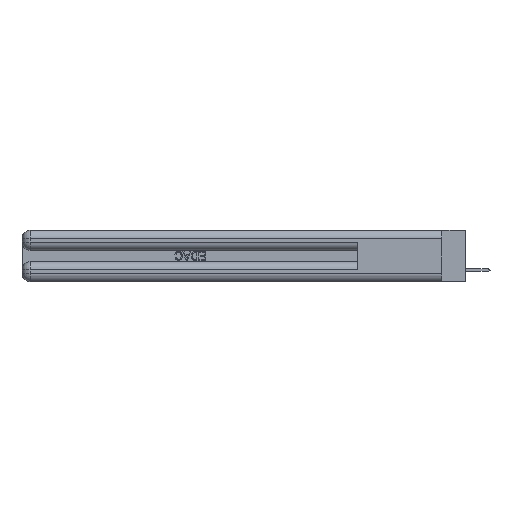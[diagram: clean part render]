
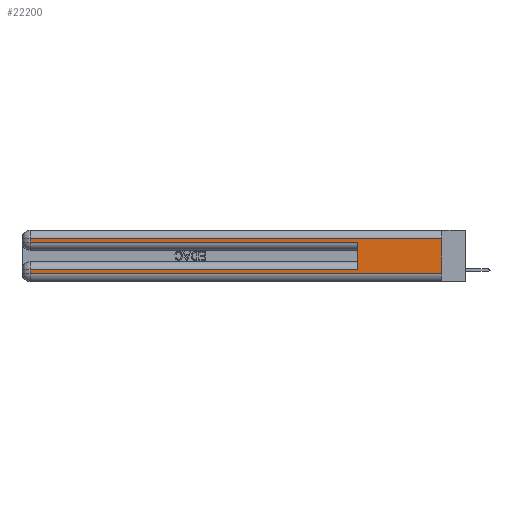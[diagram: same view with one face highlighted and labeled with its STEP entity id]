
A CAD part, left-side view. The second image highlights one B-rep face of the part: STEP entity #22200.
In plain terms, the highlighted planar face has unit normal (-1, 0, 0).
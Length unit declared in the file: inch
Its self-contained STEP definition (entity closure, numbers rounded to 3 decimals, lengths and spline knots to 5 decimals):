
#87 = EDGE_CURVE ( 'NONE', #17412, #18980, #23298, .T. ) ;
#393 = DIRECTION ( 'NONE',  ( 0., -1., 0. ) ) ;
#1524 = DIRECTION ( 'NONE',  ( 0., 0., -1. ) ) ;
#2635 = FACE_OUTER_BOUND ( 'NONE', #38131, .T. ) ;
#3554 = LINE ( 'NONE', #44252, #30137 ) ;
#4403 = LINE ( 'NONE', #26620, #36100 ) ;
#4473 = ORIENTED_EDGE ( 'NONE', *, *, #4612, .T. ) ;
#4612 = EDGE_CURVE ( 'NONE', #8973, #6380, #8666, .T. ) ;
#4940 = EDGE_CURVE ( 'NONE', #36621, #8973, #3554, .T. ) ;
#5644 = ORIENTED_EDGE ( 'NONE', *, *, #29355, .T. ) ;
#6380 = VERTEX_POINT ( 'NONE', #15923 ) ;
#6638 = LINE ( 'NONE', #37031, #34373 ) ;
#8666 = LINE ( 'NONE', #25550, #30186 ) ;
#8712 = ORIENTED_EDGE ( 'NONE', *, *, #26501, .T. ) ;
#8973 = VERTEX_POINT ( 'NONE', #36104 ) ;
#9249 = VERTEX_POINT ( 'NONE', #35643 ) ;
#11615 = CARTESIAN_POINT ( 'NONE',  ( 0., 2.94, 0.085 ) ) ;
#12524 = DIRECTION ( 'NONE',  ( 0., 0., -1. ) ) ;
#12694 = DIRECTION ( 'NONE',  ( 0., 0., -1. ) ) ;
#13653 = VECTOR ( 'NONE', #31920, 39.37008 ) ;
#13736 = VECTOR ( 'NONE', #12694, 39.37008 ) ;
#14757 = VECTOR ( 'NONE', #45902, 39.37008 ) ;
#14992 = ORIENTED_EDGE ( 'NONE', *, *, #45165, .T. ) ;
#15343 = LINE ( 'NONE', #33871, #14757 ) ;
#15381 = CARTESIAN_POINT ( 'NONE',  ( 0., 0., 0.06 ) ) ;
#15923 = CARTESIAN_POINT ( 'NONE',  ( 0., 0.6, 0.285 ) ) ;
#16619 = AXIS2_PLACEMENT_3D ( 'NONE', #26247, #44948, #12524 ) ;
#17412 = VERTEX_POINT ( 'NONE', #37823 ) ;
#18142 = LINE ( 'NONE', #28264, #13653 ) ;
#18980 = VERTEX_POINT ( 'NONE', #15381 ) ;
#19995 = ORIENTED_EDGE ( 'NONE', *, *, #45039, .F. ) ;
#21634 = ORIENTED_EDGE ( 'NONE', *, *, #87, .F. ) ;
#22200 = ADVANCED_FACE ( 'NONE', ( #2635 ), #25349, .F. ) ;
#23298 = LINE ( 'NONE', #44795, #13736 ) ;
#23429 = DIRECTION ( 'NONE',  ( 0., 0., 1. ) ) ;
#25224 = EDGE_CURVE ( 'NONE', #9249, #36015, #18142, .T. ) ;
#25349 = PLANE ( 'NONE',  #16619 ) ;
#25550 = CARTESIAN_POINT ( 'NONE',  ( 0., 0., 0.285 ) ) ;
#26247 = CARTESIAN_POINT ( 'NONE',  ( 0., 0., 0.37 ) ) ;
#26501 = EDGE_CURVE ( 'NONE', #17412, #36621, #15343, .T. ) ;
#26620 = CARTESIAN_POINT ( 'NONE',  ( 0., 0., 0.06 ) ) ;
#26859 = ORIENTED_EDGE ( 'NONE', *, *, #25224, .T. ) ;
#28264 = CARTESIAN_POINT ( 'NONE',  ( 0., 0., 0.085 ) ) ;
#29355 = EDGE_CURVE ( 'NONE', #43444, #18980, #4403, .T. ) ;
#29929 = DIRECTION ( 'NONE',  ( 0., 0., -1. ) ) ;
#30137 = VECTOR ( 'NONE', #1524, 39.37008 ) ;
#30186 = VECTOR ( 'NONE', #36624, 39.37008 ) ;
#30330 = ORIENTED_EDGE ( 'NONE', *, *, #4940, .T. ) ;
#31920 = DIRECTION ( 'NONE',  ( 0., 1., 0. ) ) ;
#33871 = CARTESIAN_POINT ( 'NONE',  ( 0., 0., 0.31 ) ) ;
#34373 = VECTOR ( 'NONE', #29929, 39.37008 ) ;
#35643 = CARTESIAN_POINT ( 'NONE',  ( 0., 0.6, 0.085 ) ) ;
#36015 = VERTEX_POINT ( 'NONE', #11615 ) ;
#36100 = VECTOR ( 'NONE', #393, 39.37008 ) ;
#36104 = CARTESIAN_POINT ( 'NONE',  ( 0., 2.94, 0.285 ) ) ;
#36621 = VERTEX_POINT ( 'NONE', #44318 ) ;
#36624 = DIRECTION ( 'NONE',  ( 0., -1., 0. ) ) ;
#37031 = CARTESIAN_POINT ( 'NONE',  ( 0., 2.94, 0.37 ) ) ;
#37249 = CARTESIAN_POINT ( 'NONE',  ( 0., 2.94, 0.06 ) ) ;
#37823 = CARTESIAN_POINT ( 'NONE',  ( 0., 0., 0.31 ) ) ;
#38131 = EDGE_LOOP ( 'NONE', ( #21634, #8712, #30330, #4473, #19995, #26859, #14992, #5644 ) ) ;
#41532 = CARTESIAN_POINT ( 'NONE',  ( 0., 0.6, 0.145 ) ) ;
#41704 = VECTOR ( 'NONE', #23429, 39.37008 ) ;
#43444 = VERTEX_POINT ( 'NONE', #37249 ) ;
#44252 = CARTESIAN_POINT ( 'NONE',  ( 0., 2.94, 0.37 ) ) ;
#44318 = CARTESIAN_POINT ( 'NONE',  ( 0., 2.94, 0.31 ) ) ;
#44795 = CARTESIAN_POINT ( 'NONE',  ( 0., 0., 0.37 ) ) ;
#44948 = DIRECTION ( 'NONE',  ( 1., 0., 0. ) ) ;
#45039 = EDGE_CURVE ( 'NONE', #9249, #6380, #46825, .T. ) ;
#45165 = EDGE_CURVE ( 'NONE', #36015, #43444, #6638, .T. ) ;
#45902 = DIRECTION ( 'NONE',  ( 0., 1., 0. ) ) ;
#46825 = LINE ( 'NONE', #41532, #41704 ) ;
